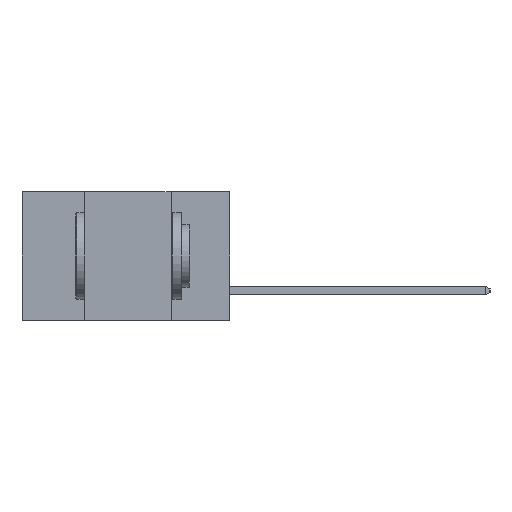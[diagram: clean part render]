
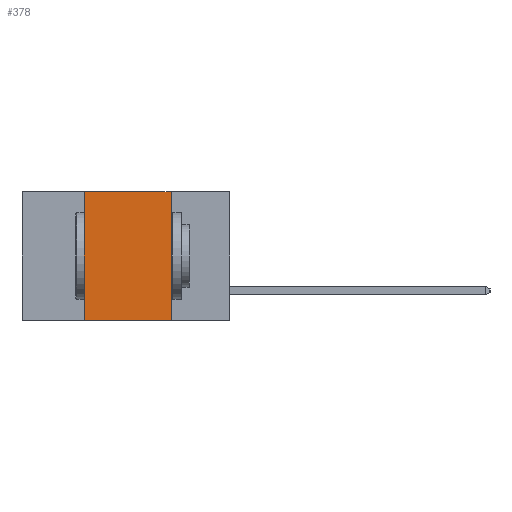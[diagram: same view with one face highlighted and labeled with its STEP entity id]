
A CAD part, left-side view. The second image highlights one B-rep face of the part: STEP entity #378.
In plain terms, the highlighted planar face has unit normal (-1, 0, 0).
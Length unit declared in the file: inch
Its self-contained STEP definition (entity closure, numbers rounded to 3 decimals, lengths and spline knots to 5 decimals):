
#64 = CARTESIAN_POINT ( 'NONE',  ( 0., 0.6, -0.37 ) ) ;
#136 = CARTESIAN_POINT ( 'NONE',  ( 0., 0.17, 0. ) ) ;
#185 = ORIENTED_EDGE ( 'NONE', *, *, #8720, .F. ) ;
#299 = CARTESIAN_POINT ( 'NONE',  ( 0., 0.6, 0. ) ) ;
#378 = ADVANCED_FACE ( 'NONE', ( #10669 ), #7422, .F. ) ;
#399 = CARTESIAN_POINT ( 'NONE',  ( 0., 0.17, -0.37 ) ) ;
#1018 = CARTESIAN_POINT ( 'NONE',  ( 0., 0.42, -0.37 ) ) ;
#1190 = AXIS2_PLACEMENT_3D ( 'NONE', #9194, #2074, #10520 ) ;
#1421 = LINE ( 'NONE', #299, #10730 ) ;
#1473 = LINE ( 'NONE', #136, #8192 ) ;
#1559 = EDGE_CURVE ( 'NONE', #9636, #8967, #1473, .T. ) ;
#2068 = EDGE_LOOP ( 'NONE', ( #4251, #11685, #185, #2855 ) ) ;
#2074 = DIRECTION ( 'NONE',  ( 1., 0., 0. ) ) ;
#2855 = ORIENTED_EDGE ( 'NONE', *, *, #4960, .T. ) ;
#3012 = DIRECTION ( 'NONE',  ( 0., 0., 1. ) ) ;
#4251 = ORIENTED_EDGE ( 'NONE', *, *, #1559, .F. ) ;
#4960 = EDGE_CURVE ( 'NONE', #10628, #8967, #5327, .T. ) ;
#5192 = VERTEX_POINT ( 'NONE', #10150 ) ;
#5327 = LINE ( 'NONE', #64, #11662 ) ;
#5943 = DIRECTION ( 'NONE',  ( 0., 0., -1. ) ) ;
#6961 = LINE ( 'NONE', #10065, #9000 ) ;
#7422 = PLANE ( 'NONE',  #1190 ) ;
#8192 = VECTOR ( 'NONE', #5943, 39.37008 ) ;
#8609 = DIRECTION ( 'NONE',  ( 0., -1., 0. ) ) ;
#8681 = CARTESIAN_POINT ( 'NONE',  ( 0., 0.17, 0. ) ) ;
#8720 = EDGE_CURVE ( 'NONE', #10628, #5192, #6961, .T. ) ;
#8967 = VERTEX_POINT ( 'NONE', #399 ) ;
#9000 = VECTOR ( 'NONE', #3012, 39.37008 ) ;
#9194 = CARTESIAN_POINT ( 'NONE',  ( 0., 0.6, 0. ) ) ;
#9590 = EDGE_CURVE ( 'NONE', #5192, #9636, #1421, .T. ) ;
#9636 = VERTEX_POINT ( 'NONE', #8681 ) ;
#10065 = CARTESIAN_POINT ( 'NONE',  ( 0., 0.42, 0. ) ) ;
#10150 = CARTESIAN_POINT ( 'NONE',  ( 0., 0.42, 0. ) ) ;
#10520 = DIRECTION ( 'NONE',  ( 0., 0., -1. ) ) ;
#10592 = DIRECTION ( 'NONE',  ( 0., -1., 0. ) ) ;
#10628 = VERTEX_POINT ( 'NONE', #1018 ) ;
#10669 = FACE_OUTER_BOUND ( 'NONE', #2068, .T. ) ;
#10730 = VECTOR ( 'NONE', #8609, 39.37008 ) ;
#11662 = VECTOR ( 'NONE', #10592, 39.37008 ) ;
#11685 = ORIENTED_EDGE ( 'NONE', *, *, #9590, .F. ) ;
